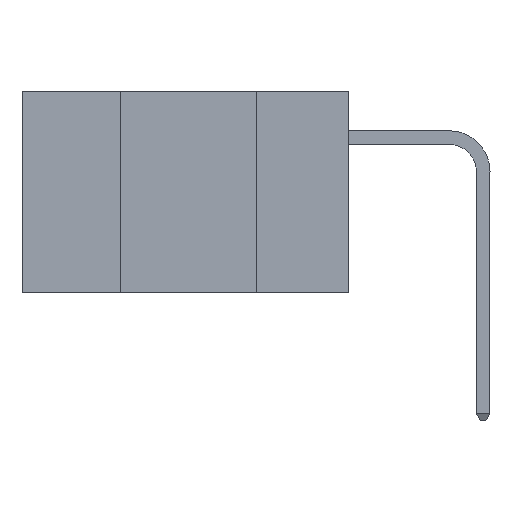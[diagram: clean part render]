
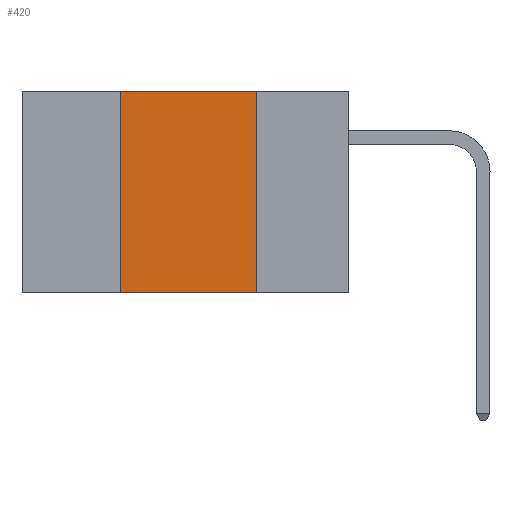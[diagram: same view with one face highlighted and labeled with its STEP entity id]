
A CAD part, left-side view. The second image highlights one B-rep face of the part: STEP entity #420.
In plain terms, the highlighted planar face has unit normal (-1, 0, 0).
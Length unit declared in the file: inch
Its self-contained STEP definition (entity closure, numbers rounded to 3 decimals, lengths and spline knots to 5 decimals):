
#420 = ADVANCED_FACE ( 'NONE', ( #35648 ), #2515, .F. ) ;
#1585 = ORIENTED_EDGE ( 'NONE', *, *, #29117, .T. ) ;
#2515 = PLANE ( 'NONE',  #19873 ) ;
#3390 = CARTESIAN_POINT ( 'NONE',  ( 0., 0.17, -0.37 ) ) ;
#3554 = VECTOR ( 'NONE', #31751, 39.37008 ) ;
#4452 = CARTESIAN_POINT ( 'NONE',  ( 0., 0.17, 0. ) ) ;
#4818 = LINE ( 'NONE', #9672, #34657 ) ;
#5360 = CARTESIAN_POINT ( 'NONE',  ( 0., 0.6, 0. ) ) ;
#6096 = EDGE_CURVE ( 'NONE', #6462, #29389, #21968, .T. ) ;
#6462 = VERTEX_POINT ( 'NONE', #35240 ) ;
#8283 = DIRECTION ( 'NONE',  ( 1., 0., 0. ) ) ;
#9672 = CARTESIAN_POINT ( 'NONE',  ( 0., 0.6, -0.37 ) ) ;
#10148 = VERTEX_POINT ( 'NONE', #28228 ) ;
#12480 = VECTOR ( 'NONE', #28750, 39.37008 ) ;
#14327 = VECTOR ( 'NONE', #16465, 39.37008 ) ;
#15170 = EDGE_LOOP ( 'NONE', ( #24268, #22552, #18078, #1585 ) ) ;
#16465 = DIRECTION ( 'NONE',  ( 0., -1., 0. ) ) ;
#18078 = ORIENTED_EDGE ( 'NONE', *, *, #30349, .F. ) ;
#19873 = AXIS2_PLACEMENT_3D ( 'NONE', #5360, #8283, #28468 ) ;
#21968 = LINE ( 'NONE', #22094, #14327 ) ;
#22094 = CARTESIAN_POINT ( 'NONE',  ( 0., 0.6, 0. ) ) ;
#22552 = ORIENTED_EDGE ( 'NONE', *, *, #6096, .F. ) ;
#24059 = DIRECTION ( 'NONE',  ( 0., -1., 0. ) ) ;
#24268 = ORIENTED_EDGE ( 'NONE', *, *, #33539, .F. ) ;
#24828 = LINE ( 'NONE', #28826, #3554 ) ;
#28228 = CARTESIAN_POINT ( 'NONE',  ( 0., 0.42, -0.37 ) ) ;
#28376 = VERTEX_POINT ( 'NONE', #3390 ) ;
#28468 = DIRECTION ( 'NONE',  ( 0., 0., -1. ) ) ;
#28750 = DIRECTION ( 'NONE',  ( 0., 0., 1. ) ) ;
#28826 = CARTESIAN_POINT ( 'NONE',  ( 0., 0.17, 0. ) ) ;
#29117 = EDGE_CURVE ( 'NONE', #10148, #28376, #4818, .T. ) ;
#29389 = VERTEX_POINT ( 'NONE', #4452 ) ;
#30349 = EDGE_CURVE ( 'NONE', #10148, #6462, #36329, .T. ) ;
#31751 = DIRECTION ( 'NONE',  ( 0., 0., -1. ) ) ;
#33539 = EDGE_CURVE ( 'NONE', #29389, #28376, #24828, .T. ) ;
#34615 = CARTESIAN_POINT ( 'NONE',  ( 0., 0.42, 0. ) ) ;
#34657 = VECTOR ( 'NONE', #24059, 39.37008 ) ;
#35240 = CARTESIAN_POINT ( 'NONE',  ( 0., 0.42, 0. ) ) ;
#35648 = FACE_OUTER_BOUND ( 'NONE', #15170, .T. ) ;
#36329 = LINE ( 'NONE', #34615, #12480 ) ;
